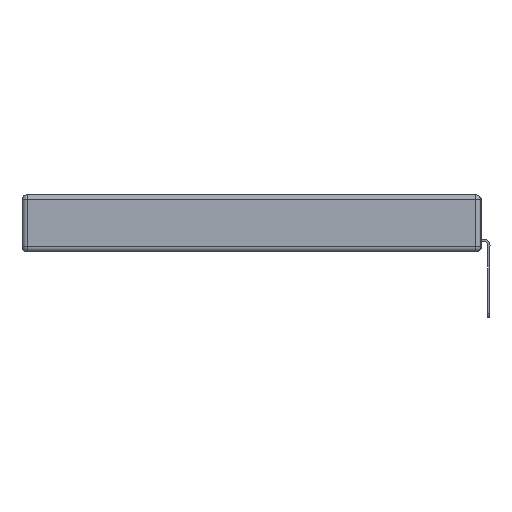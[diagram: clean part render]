
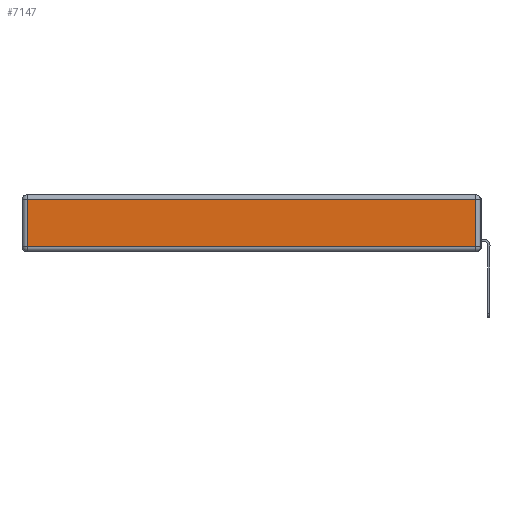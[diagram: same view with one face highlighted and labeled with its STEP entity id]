
A CAD part, left-side view. The second image highlights one B-rep face of the part: STEP entity #7147.
In plain terms, the highlighted planar face has unit normal (-1, 0, 0).
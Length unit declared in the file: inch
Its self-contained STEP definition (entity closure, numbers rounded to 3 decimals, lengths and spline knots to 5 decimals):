
#51 = EDGE_CURVE ( 'NONE', #7668, #20156, #9531, .T. ) ;
#1715 = DIRECTION ( 'NONE',  ( 0., 0., -1. ) ) ;
#2361 = FACE_OUTER_BOUND ( 'NONE', #7275, .T. ) ;
#3265 = CARTESIAN_POINT ( 'NONE',  ( 0., 2.75, -0.03 ) ) ;
#3689 = ORIENTED_EDGE ( 'NONE', *, *, #15348, .T. ) ;
#3865 = ORIENTED_EDGE ( 'NONE', *, *, #8500, .T. ) ;
#4209 = CARTESIAN_POINT ( 'NONE',  ( 0., 2.72, -0.313 ) ) ;
#4562 = VECTOR ( 'NONE', #10128, 39.37008 ) ;
#4999 = DIRECTION ( 'NONE',  ( 0., 1., 0. ) ) ;
#7147 = ADVANCED_FACE ( 'NONE', ( #2361 ), #7972, .T. ) ;
#7275 = EDGE_LOOP ( 'NONE', ( #12384, #3865, #18739, #3689 ) ) ;
#7373 = LINE ( 'NONE', #3265, #22316 ) ;
#7668 = VERTEX_POINT ( 'NONE', #4209 ) ;
#7972 = PLANE ( 'NONE',  #17181 ) ;
#8135 = LINE ( 'NONE', #11153, #16668 ) ;
#8470 = CARTESIAN_POINT ( 'NONE',  ( 0., 2.72, -0.03 ) ) ;
#8500 = EDGE_CURVE ( 'NONE', #20156, #21806, #8135, .T. ) ;
#8985 = VECTOR ( 'NONE', #1715, 39.37008 ) ;
#9334 = DIRECTION ( 'NONE',  ( 0., 0., 1. ) ) ;
#9531 = LINE ( 'NONE', #11882, #4562 ) ;
#9560 = LINE ( 'NONE', #12938, #8985 ) ;
#9584 = VERTEX_POINT ( 'NONE', #8470 ) ;
#9707 = DIRECTION ( 'NONE',  ( -1., 0., 0. ) ) ;
#10128 = DIRECTION ( 'NONE',  ( 0., -1., 0. ) ) ;
#11153 = CARTESIAN_POINT ( 'NONE',  ( 0., 0.03, -0.343 ) ) ;
#11882 = CARTESIAN_POINT ( 'NONE',  ( 0., 0., -0.313 ) ) ;
#12384 = ORIENTED_EDGE ( 'NONE', *, *, #51, .T. ) ;
#12938 = CARTESIAN_POINT ( 'NONE',  ( 0., 2.72, -0.343 ) ) ;
#15348 = EDGE_CURVE ( 'NONE', #9584, #7668, #9560, .T. ) ;
#15708 = CARTESIAN_POINT ( 'NONE',  ( 0., 0., -0.343 ) ) ;
#16668 = VECTOR ( 'NONE', #9334, 39.37008 ) ;
#17181 = AXIS2_PLACEMENT_3D ( 'NONE', #15708, #9707, #21094 ) ;
#18739 = ORIENTED_EDGE ( 'NONE', *, *, #20166, .T. ) ;
#18906 = CARTESIAN_POINT ( 'NONE',  ( 0., 0.03, -0.03 ) ) ;
#20057 = CARTESIAN_POINT ( 'NONE',  ( 0., 0.03, -0.313 ) ) ;
#20156 = VERTEX_POINT ( 'NONE', #20057 ) ;
#20166 = EDGE_CURVE ( 'NONE', #21806, #9584, #7373, .T. ) ;
#21094 = DIRECTION ( 'NONE',  ( 0., 0., 1. ) ) ;
#21806 = VERTEX_POINT ( 'NONE', #18906 ) ;
#22316 = VECTOR ( 'NONE', #4999, 39.37008 ) ;
